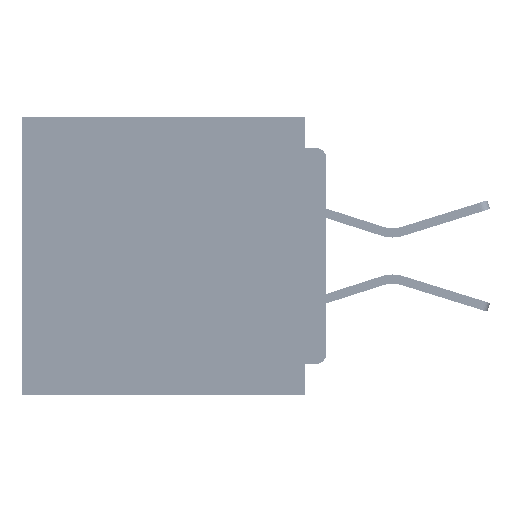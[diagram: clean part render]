
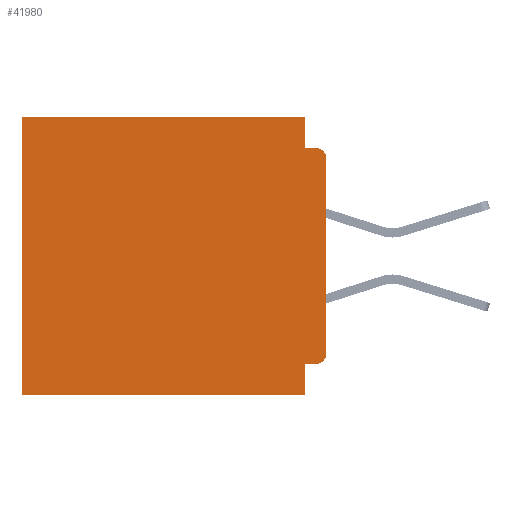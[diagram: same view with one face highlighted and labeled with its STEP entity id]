
A CAD part, left-side view. The second image highlights one B-rep face of the part: STEP entity #41980.
In plain terms, the highlighted planar face has unit normal (-1, 0, 0).
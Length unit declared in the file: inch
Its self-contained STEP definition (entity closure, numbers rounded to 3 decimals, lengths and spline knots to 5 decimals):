
#628 = VECTOR ( 'NONE', #44741, 39.37008 ) ;
#2026 = LINE ( 'NONE', #51520, #55423 ) ;
#2343 = VECTOR ( 'NONE', #21141, 39.37008 ) ;
#2371 = CARTESIAN_POINT ( 'NONE',  ( 0.3, 0., -0.06 ) ) ;
#4060 = ORIENTED_EDGE ( 'NONE', *, *, #26755, .F. ) ;
#4139 = ORIENTED_EDGE ( 'NONE', *, *, #24076, .T. ) ;
#4373 = CARTESIAN_POINT ( 'NONE',  ( 0.3, 0.015, -0.045 ) ) ;
#5176 = CARTESIAN_POINT ( 'NONE',  ( 0.3, 0.031, -0.355 ) ) ;
#5299 = EDGE_CURVE ( 'NONE', #53620, #55013, #61229, .T. ) ;
#5681 = CARTESIAN_POINT ( 'NONE',  ( 0.3, 0.437, -0.4 ) ) ;
#5713 = CIRCLE ( 'NONE', #42007, 0.015 ) ;
#6063 = DIRECTION ( 'NONE',  ( -1., 0., 0. ) ) ;
#7013 = PLANE ( 'NONE',  #11604 ) ;
#7346 = DIRECTION ( 'NONE',  ( 0., 1., 0. ) ) ;
#7505 = VERTEX_POINT ( 'NONE', #5176 ) ;
#8132 = ORIENTED_EDGE ( 'NONE', *, *, #5299, .F. ) ;
#8953 = ORIENTED_EDGE ( 'NONE', *, *, #62930, .T. ) ;
#9814 = EDGE_LOOP ( 'NONE', ( #37252, #8953, #56657, #8132, #63046, #4139, #21867, #4060, #34880, #53388 ) ) ;
#11604 = AXIS2_PLACEMENT_3D ( 'NONE', #48341, #17462, #53591 ) ;
#13743 = CARTESIAN_POINT ( 'NONE',  ( 0.3, 0.031, 0. ) ) ;
#14156 = CIRCLE ( 'NONE', #30180, 0.015 ) ;
#14385 = LINE ( 'NONE', #49711, #628 ) ;
#16079 = VERTEX_POINT ( 'NONE', #51835 ) ;
#16371 = LINE ( 'NONE', #25435, #43815 ) ;
#17309 = EDGE_CURVE ( 'NONE', #32420, #37396, #23866, .T. ) ;
#17462 = DIRECTION ( 'NONE',  ( 1., 0., 0. ) ) ;
#17551 = CARTESIAN_POINT ( 'NONE',  ( 0.3, 0., 0. ) ) ;
#19145 = EDGE_CURVE ( 'NONE', #62152, #7505, #16371, .T. ) ;
#20058 = EDGE_CURVE ( 'NONE', #62152, #16079, #14156, .T. ) ;
#21141 = DIRECTION ( 'NONE',  ( 0., 0., -1. ) ) ;
#21867 = ORIENTED_EDGE ( 'NONE', *, *, #17309, .F. ) ;
#22375 = DIRECTION ( 'NONE',  ( -1., 0., 0. ) ) ;
#23866 = LINE ( 'NONE', #36836, #34384 ) ;
#24076 = EDGE_CURVE ( 'NONE', #38117, #37396, #57329, .T. ) ;
#25222 = CARTESIAN_POINT ( 'NONE',  ( 0.3, 0.015, -0.355 ) ) ;
#25435 = CARTESIAN_POINT ( 'NONE',  ( 0.3, 0., -0.355 ) ) ;
#26330 = LINE ( 'NONE', #62943, #38441 ) ;
#26755 = EDGE_CURVE ( 'NONE', #7505, #32420, #26330, .T. ) ;
#29516 = CARTESIAN_POINT ( 'NONE',  ( 0.3, 0.031, -0.045 ) ) ;
#30075 = FACE_OUTER_BOUND ( 'NONE', #9814, .T. ) ;
#30180 = AXIS2_PLACEMENT_3D ( 'NONE', #53286, #22375, #58444 ) ;
#30648 = DIRECTION ( 'NONE',  ( 0., 1., 0. ) ) ;
#30755 = CARTESIAN_POINT ( 'NONE',  ( 0.3, 0.437, 0. ) ) ;
#31030 = DIRECTION ( 'NONE',  ( 0., -1., 0. ) ) ;
#32420 = VERTEX_POINT ( 'NONE', #55564 ) ;
#32879 = VERTEX_POINT ( 'NONE', #2371 ) ;
#34384 = VECTOR ( 'NONE', #52356, 39.37008 ) ;
#34880 = ORIENTED_EDGE ( 'NONE', *, *, #19145, .F. ) ;
#36836 = CARTESIAN_POINT ( 'NONE',  ( 0.3, 0., -0.4 ) ) ;
#37098 = CARTESIAN_POINT ( 'NONE',  ( 0.3, 0.015, -0.06 ) ) ;
#37252 = ORIENTED_EDGE ( 'NONE', *, *, #53689, .F. ) ;
#37396 = VERTEX_POINT ( 'NONE', #43357 ) ;
#37622 = EDGE_CURVE ( 'NONE', #55013, #49763, #2026, .T. ) ;
#38117 = VERTEX_POINT ( 'NONE', #30755 ) ;
#38441 = VECTOR ( 'NONE', #42464, 39.37008 ) ;
#39354 = CARTESIAN_POINT ( 'NONE',  ( 0.3, 0.031, 0. ) ) ;
#39736 = VECTOR ( 'NONE', #7346, 39.37008 ) ;
#41980 = ADVANCED_FACE ( 'NONE', ( #30075 ), #7013, .F. ) ;
#42007 = AXIS2_PLACEMENT_3D ( 'NONE', #37098, #6063, #42243 ) ;
#42243 = DIRECTION ( 'NONE',  ( 0., 0., -1. ) ) ;
#42464 = DIRECTION ( 'NONE',  ( 0., 0., -1. ) ) ;
#42669 = VECTOR ( 'NONE', #65075, 39.37008 ) ;
#43357 = CARTESIAN_POINT ( 'NONE',  ( 0.3, 0.437, -0.4 ) ) ;
#43815 = VECTOR ( 'NONE', #30648, 39.37008 ) ;
#44741 = DIRECTION ( 'NONE',  ( 0., 0., -1. ) ) ;
#48341 = CARTESIAN_POINT ( 'NONE',  ( 0.3, 0., -0.4 ) ) ;
#48527 = EDGE_CURVE ( 'NONE', #53620, #38117, #53436, .T. ) ;
#49711 = CARTESIAN_POINT ( 'NONE',  ( 0.3, 0., -0.4 ) ) ;
#49763 = VERTEX_POINT ( 'NONE', #4373 ) ;
#51520 = CARTESIAN_POINT ( 'NONE',  ( 0.3, 0., -0.045 ) ) ;
#51835 = CARTESIAN_POINT ( 'NONE',  ( 0.3, 0., -0.34 ) ) ;
#52356 = DIRECTION ( 'NONE',  ( 0., 1., 0. ) ) ;
#53286 = CARTESIAN_POINT ( 'NONE',  ( 0.3, 0.015, -0.34 ) ) ;
#53388 = ORIENTED_EDGE ( 'NONE', *, *, #20058, .T. ) ;
#53436 = LINE ( 'NONE', #17551, #39736 ) ;
#53591 = DIRECTION ( 'NONE',  ( 0., 0., -1. ) ) ;
#53620 = VERTEX_POINT ( 'NONE', #39354 ) ;
#53689 = EDGE_CURVE ( 'NONE', #32879, #16079, #14385, .T. ) ;
#55013 = VERTEX_POINT ( 'NONE', #29516 ) ;
#55423 = VECTOR ( 'NONE', #31030, 39.37008 ) ;
#55564 = CARTESIAN_POINT ( 'NONE',  ( 0.3, 0.031, -0.4 ) ) ;
#56657 = ORIENTED_EDGE ( 'NONE', *, *, #37622, .F. ) ;
#57329 = LINE ( 'NONE', #5681, #2343 ) ;
#58444 = DIRECTION ( 'NONE',  ( 0., 0., -1. ) ) ;
#61229 = LINE ( 'NONE', #13743, #42669 ) ;
#62152 = VERTEX_POINT ( 'NONE', #25222 ) ;
#62930 = EDGE_CURVE ( 'NONE', #32879, #49763, #5713, .T. ) ;
#62943 = CARTESIAN_POINT ( 'NONE',  ( 0.3, 0.031, -0.4 ) ) ;
#63046 = ORIENTED_EDGE ( 'NONE', *, *, #48527, .T. ) ;
#65075 = DIRECTION ( 'NONE',  ( 0., 0., -1. ) ) ;
